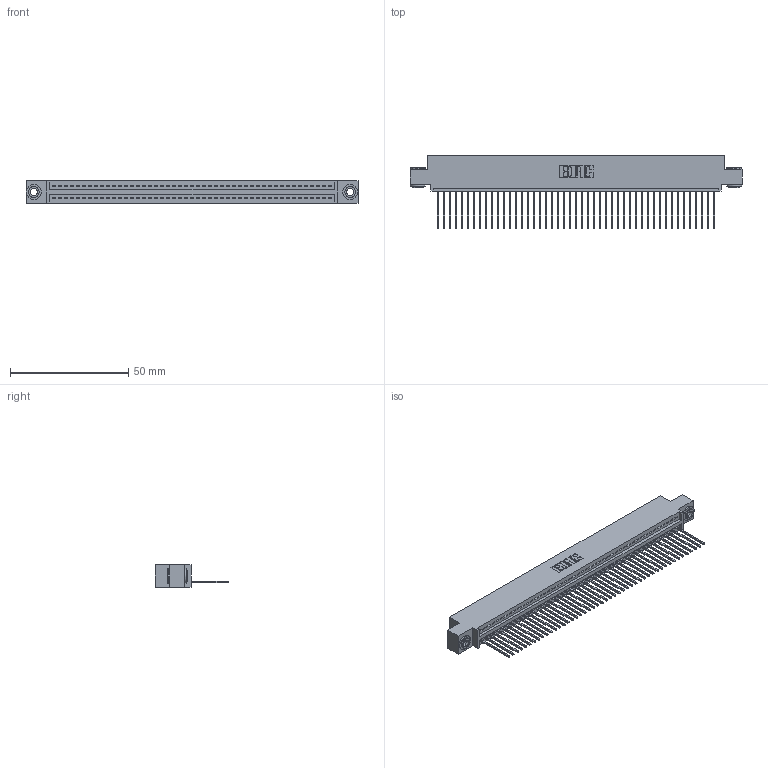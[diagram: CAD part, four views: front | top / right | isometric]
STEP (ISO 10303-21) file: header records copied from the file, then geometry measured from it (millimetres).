
FILE_DESCRIPTION (( 'STEP AP203' ), '1' );
FILE_NAME ('345-047-542-403.STEP', '2019-10-09T02:57:51', ( '' ), ( '' ), 'SwSTEP 2.0', 'SolidWorks 2016', '' );
FILE_SCHEMA (( 'CONFIG_CONTROL_DESIGN' ));
Length unit declared in the file: inch
Products named in the file (4): 345-292-001_345-293-142; 345-047-542-403; 345-250-002_345-250-002-102; 345 Part_0.110 Offset - 0.156 Dia-TH
Assembly tree (50 placements, depth 2):
  345-047-542-403
    345 Part_0.110 Offset - 0.156 Dia-TH
    345-292-001_345-293-142  x47
    345-250-002_345-250-002-102  x2
Bounding box: 140.59 x 31.29 x 9.4 mm (x, y, z)
Volume: 13444.8 mm3; surface area: 18892.6 mm2
Topology: 50 solids, 50 shells, 2894 faces, 8701 edges, 5734 vertices
Faces by surface type: plane 1974, cylinder 912, cone 8
Entity records: 35500 total; most frequent: CARTESIAN_POINT 6128, ORIENTED_EDGE 6102, DIRECTION 5375, EDGE_CURVE 3051, LINE 2707, VECTOR 2707, VERTEX_POINT 2030, AXIS2_PLACEMENT_3D 1334
